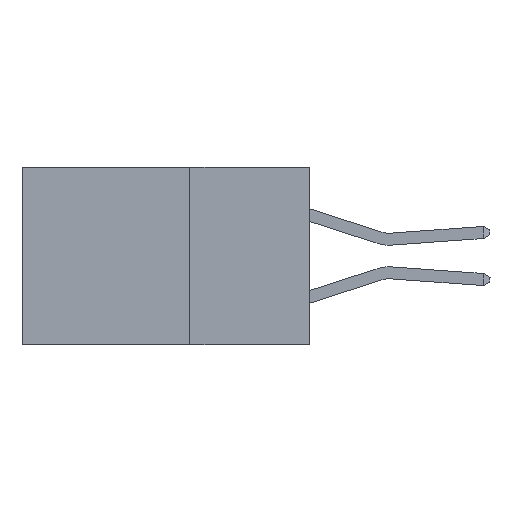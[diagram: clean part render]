
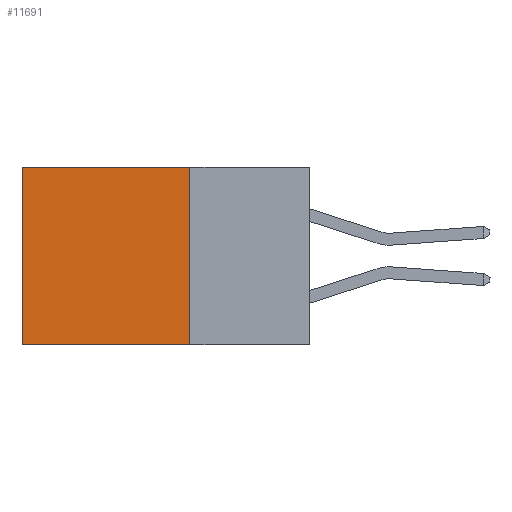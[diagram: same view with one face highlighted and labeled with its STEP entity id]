
A CAD part, left-side view. The second image highlights one B-rep face of the part: STEP entity #11691.
In plain terms, the highlighted planar face has unit normal (-1, 0, 0).
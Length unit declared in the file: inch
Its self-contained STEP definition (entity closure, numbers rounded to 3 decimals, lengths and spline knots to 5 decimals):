
#190 = AXIS2_PLACEMENT_3D ( 'NONE', #19363, #3150, #17406 ) ;
#722 = CARTESIAN_POINT ( 'NONE',  ( 0.2615, 0.25, 0. ) ) ;
#1021 = PLANE ( 'NONE',  #190 ) ;
#2156 = VERTEX_POINT ( 'NONE', #722 ) ;
#2630 = CARTESIAN_POINT ( 'NONE',  ( 0.2615, 0.25, -0.37 ) ) ;
#3027 = LINE ( 'NONE', #15209, #7897 ) ;
#3150 = DIRECTION ( 'NONE',  ( 1., 0., 0. ) ) ;
#3240 = CARTESIAN_POINT ( 'NONE',  ( 0.2615, 0.6, -0.37 ) ) ;
#3422 = ORIENTED_EDGE ( 'NONE', *, *, #15557, .F. ) ;
#3886 = LINE ( 'NONE', #2630, #14196 ) ;
#4717 = VERTEX_POINT ( 'NONE', #10638 ) ;
#5309 = EDGE_LOOP ( 'NONE', ( #25531, #12752, #3422, #22893 ) ) ;
#7897 = VECTOR ( 'NONE', #17186, 39.37008 ) ;
#10026 = LINE ( 'NONE', #11574, #11323 ) ;
#10638 = CARTESIAN_POINT ( 'NONE',  ( 0.2615, 0.25, -0.37 ) ) ;
#11323 = VECTOR ( 'NONE', #25461, 39.37008 ) ;
#11574 = CARTESIAN_POINT ( 'NONE',  ( 0.2615, 0.25, -0.37 ) ) ;
#11691 = ADVANCED_FACE ( 'NONE', ( #24399 ), #1021, .F. ) ;
#12752 = ORIENTED_EDGE ( 'NONE', *, *, #20202, .F. ) ;
#13086 = DIRECTION ( 'NONE',  ( 0., 1., 0. ) ) ;
#14196 = VECTOR ( 'NONE', #20971, 39.37008 ) ;
#14242 = EDGE_CURVE ( 'NONE', #2156, #25126, #14939, .T. ) ;
#14939 = LINE ( 'NONE', #17035, #19624 ) ;
#15209 = CARTESIAN_POINT ( 'NONE',  ( 0.2615, 0.6, -0.37 ) ) ;
#15557 = EDGE_CURVE ( 'NONE', #2156, #4717, #10026, .T. ) ;
#17035 = CARTESIAN_POINT ( 'NONE',  ( 0.2615, 0.25, 0. ) ) ;
#17186 = DIRECTION ( 'NONE',  ( 0., 0., -1. ) ) ;
#17406 = DIRECTION ( 'NONE',  ( 0., 0., -1. ) ) ;
#18256 = EDGE_CURVE ( 'NONE', #25126, #19090, #3027, .T. ) ;
#19090 = VERTEX_POINT ( 'NONE', #3240 ) ;
#19363 = CARTESIAN_POINT ( 'NONE',  ( 0.2615, 0.25, -0.37 ) ) ;
#19624 = VECTOR ( 'NONE', #13086, 39.37008 ) ;
#20202 = EDGE_CURVE ( 'NONE', #4717, #19090, #3886, .T. ) ;
#20971 = DIRECTION ( 'NONE',  ( 0., 1., 0. ) ) ;
#22893 = ORIENTED_EDGE ( 'NONE', *, *, #14242, .T. ) ;
#24399 = FACE_OUTER_BOUND ( 'NONE', #5309, .T. ) ;
#25126 = VERTEX_POINT ( 'NONE', #25653 ) ;
#25461 = DIRECTION ( 'NONE',  ( 0., 0., -1. ) ) ;
#25531 = ORIENTED_EDGE ( 'NONE', *, *, #18256, .T. ) ;
#25653 = CARTESIAN_POINT ( 'NONE',  ( 0.2615, 0.6, 0. ) ) ;
